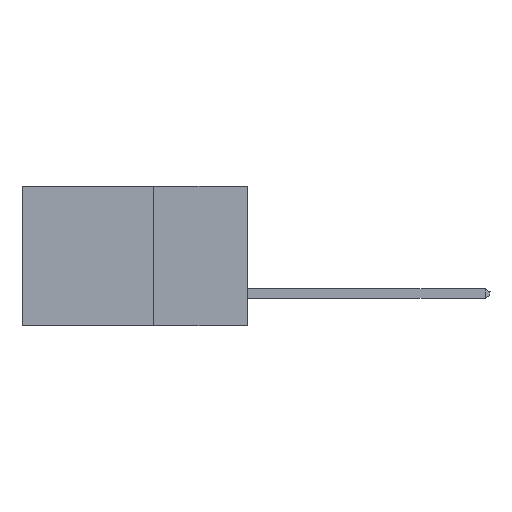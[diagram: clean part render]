
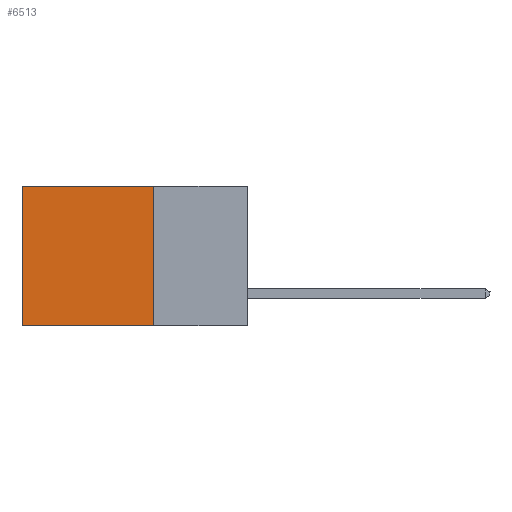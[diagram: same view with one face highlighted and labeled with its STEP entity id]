
A CAD part, left-side view. The second image highlights one B-rep face of the part: STEP entity #6513.
In plain terms, the highlighted planar face has unit normal (-1, 0, 0).
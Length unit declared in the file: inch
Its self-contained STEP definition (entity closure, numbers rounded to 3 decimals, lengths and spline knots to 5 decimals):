
#3161 = CARTESIAN_POINT ( 'NONE',  ( 0.2615, 0.25, -0.37 ) ) ;
#3182 = ORIENTED_EDGE ( 'NONE', *, *, #9644, .F. ) ;
#3713 = ORIENTED_EDGE ( 'NONE', *, *, #11845, .T. ) ;
#3743 = LINE ( 'NONE', #18920, #6210 ) ;
#3755 = CARTESIAN_POINT ( 'NONE',  ( 0.2615, 0.6, -0.37 ) ) ;
#4506 = EDGE_LOOP ( 'NONE', ( #13503, #3182, #7751, #3713 ) ) ;
#6168 = VERTEX_POINT ( 'NONE', #3161 ) ;
#6210 = VECTOR ( 'NONE', #15872, 39.37008 ) ;
#6513 = ADVANCED_FACE ( 'NONE', ( #7555 ), #12236, .F. ) ;
#7253 = CARTESIAN_POINT ( 'NONE',  ( 0.2615, 0.25, 0. ) ) ;
#7555 = FACE_OUTER_BOUND ( 'NONE', #4506, .T. ) ;
#7751 = ORIENTED_EDGE ( 'NONE', *, *, #18264, .F. ) ;
#8078 = CARTESIAN_POINT ( 'NONE',  ( 0.2615, 0.6, 0. ) ) ;
#8270 = CARTESIAN_POINT ( 'NONE',  ( 0.2615, 0.6, -0.37 ) ) ;
#9183 = VERTEX_POINT ( 'NONE', #8270 ) ;
#9644 = EDGE_CURVE ( 'NONE', #6168, #9183, #16075, .T. ) ;
#9678 = VECTOR ( 'NONE', #19652, 39.37008 ) ;
#10235 = VERTEX_POINT ( 'NONE', #8078 ) ;
#10301 = AXIS2_PLACEMENT_3D ( 'NONE', #18427, #12332, #17406 ) ;
#10314 = LINE ( 'NONE', #7253, #9678 ) ;
#11103 = CARTESIAN_POINT ( 'NONE',  ( 0.2615, 0.25, -0.37 ) ) ;
#11845 = EDGE_CURVE ( 'NONE', #12743, #10235, #10314, .T. ) ;
#12236 = PLANE ( 'NONE',  #10301 ) ;
#12332 = DIRECTION ( 'NONE',  ( 1., 0., 0. ) ) ;
#12743 = VERTEX_POINT ( 'NONE', #14084 ) ;
#13503 = ORIENTED_EDGE ( 'NONE', *, *, #18774, .T. ) ;
#14084 = CARTESIAN_POINT ( 'NONE',  ( 0.2615, 0.25, 0. ) ) ;
#14446 = DIRECTION ( 'NONE',  ( 0., 1., 0. ) ) ;
#14466 = DIRECTION ( 'NONE',  ( 0., 0., -1. ) ) ;
#15872 = DIRECTION ( 'NONE',  ( 0., 0., -1. ) ) ;
#16075 = LINE ( 'NONE', #11103, #18000 ) ;
#17273 = VECTOR ( 'NONE', #14466, 39.37008 ) ;
#17406 = DIRECTION ( 'NONE',  ( 0., 0., -1. ) ) ;
#18000 = VECTOR ( 'NONE', #14446, 39.37008 ) ;
#18264 = EDGE_CURVE ( 'NONE', #12743, #6168, #3743, .T. ) ;
#18427 = CARTESIAN_POINT ( 'NONE',  ( 0.2615, 0.25, -0.37 ) ) ;
#18774 = EDGE_CURVE ( 'NONE', #10235, #9183, #19338, .T. ) ;
#18920 = CARTESIAN_POINT ( 'NONE',  ( 0.2615, 0.25, -0.37 ) ) ;
#19338 = LINE ( 'NONE', #3755, #17273 ) ;
#19652 = DIRECTION ( 'NONE',  ( 0., 1., 0. ) ) ;
